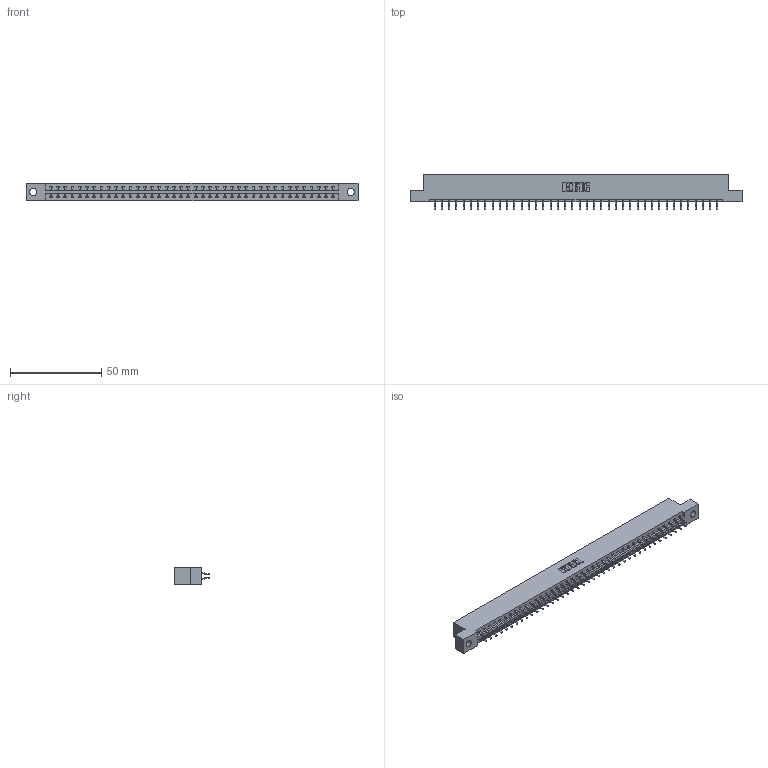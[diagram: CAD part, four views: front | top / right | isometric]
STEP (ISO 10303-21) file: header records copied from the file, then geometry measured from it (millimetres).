
FILE_DESCRIPTION (( 'STEP AP203' ), '1' );
FILE_NAME ('387-080-556-204.STEP', '2018-09-23T19:04:15', ( '' ), ( '' ), 'SwSTEP 2.0', 'SolidWorks 2016', '' );
FILE_SCHEMA (( 'CONFIG_CONTROL_DESIGN' ));
Length unit declared in the file: inch
Products named in the file (3): 337 Part_Flush Mounting Lugs - 0.156 Dia-TH; 345-292-001_556 Tail; 387-080-556-204
Assembly tree (81 placements, depth 2):
  387-080-556-204
    337 Part_Flush Mounting Lugs - 0.156 Dia-TH
    345-292-001_556 Tail  x80
Bounding box: 181.51 x 19.57 x 9.4 mm (x, y, z)
Volume: 19011.1 mm3; surface area: 21185.7 mm2
Topology: 81 solids, 81 shells, 4914 faces, 14631 edges, 9646 vertices
Faces by surface type: plane 3430, cylinder 1484
Entity records: 31495 total; most frequent: CARTESIAN_POINT 5322, ORIENTED_EDGE 5246, DIRECTION 4519, EDGE_CURVE 2623, LINE 2487, VECTOR 2487, VERTEX_POINT 1746, AXIS2_PLACEMENT_3D 1016
